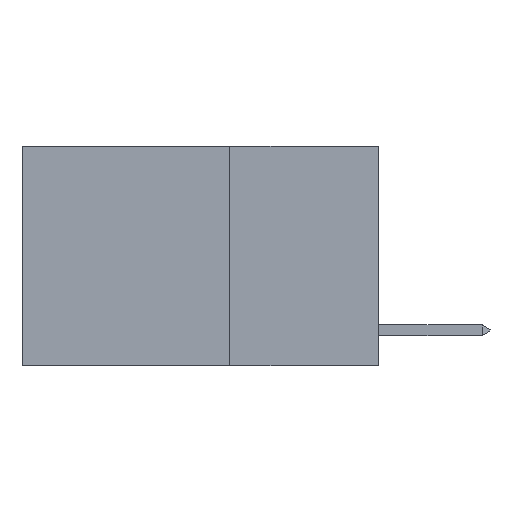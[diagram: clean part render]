
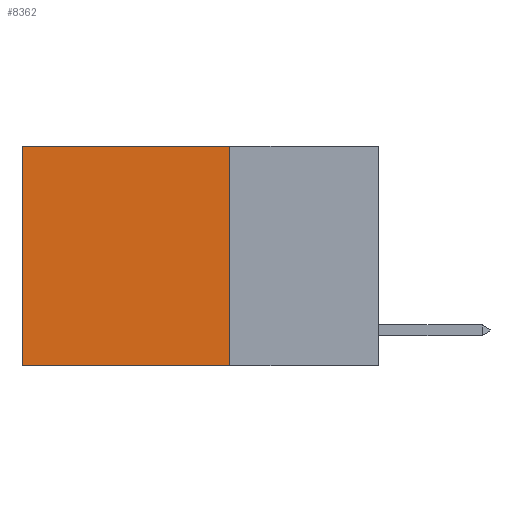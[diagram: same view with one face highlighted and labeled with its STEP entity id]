
A CAD part, left-side view. The second image highlights one B-rep face of the part: STEP entity #8362.
In plain terms, the highlighted planar face has unit normal (-1, 0, 0).
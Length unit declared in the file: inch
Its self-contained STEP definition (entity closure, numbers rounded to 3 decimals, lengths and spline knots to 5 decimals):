
#175 = VECTOR ( 'NONE', #8512, 39.37008 ) ;
#304 = EDGE_CURVE ( 'NONE', #1968, #10467, #11217, .T. ) ;
#358 = ORIENTED_EDGE ( 'NONE', *, *, #304, .F. ) ;
#713 = ORIENTED_EDGE ( 'NONE', *, *, #8503, .F. ) ;
#1292 = EDGE_CURVE ( 'NONE', #1968, #9118, #7324, .T. ) ;
#1561 = CARTESIAN_POINT ( 'NONE',  ( 0.2625, 0.25, -0.37 ) ) ;
#1917 = CARTESIAN_POINT ( 'NONE',  ( 0.2625, 0.25, 0. ) ) ;
#1968 = VERTEX_POINT ( 'NONE', #3652 ) ;
#2159 = DIRECTION ( 'NONE',  ( 0., 1., 0. ) ) ;
#2371 = VECTOR ( 'NONE', #3181, 39.37008 ) ;
#2618 = VECTOR ( 'NONE', #2159, 39.37008 ) ;
#2633 = ORIENTED_EDGE ( 'NONE', *, *, #3169, .T. ) ;
#2778 = LINE ( 'NONE', #3753, #175 ) ;
#3169 = EDGE_CURVE ( 'NONE', #9118, #8665, #2778, .T. ) ;
#3181 = DIRECTION ( 'NONE',  ( 0., 1., 0. ) ) ;
#3652 = CARTESIAN_POINT ( 'NONE',  ( 0.2625, 0.25, 0. ) ) ;
#3753 = CARTESIAN_POINT ( 'NONE',  ( 0.2625, 0.6, 0. ) ) ;
#4064 = CARTESIAN_POINT ( 'NONE',  ( 0.2625, 0.25, 0. ) ) ;
#4105 = PLANE ( 'NONE',  #7825 ) ;
#4203 = CARTESIAN_POINT ( 'NONE',  ( 0.2625, 0.25, -0.37 ) ) ;
#4768 = EDGE_LOOP ( 'NONE', ( #2633, #713, #358, #6042 ) ) ;
#5844 = DIRECTION ( 'NONE',  ( 1., 0., 0. ) ) ;
#5882 = CARTESIAN_POINT ( 'NONE',  ( 0.2625, 0.6, 0. ) ) ;
#6042 = ORIENTED_EDGE ( 'NONE', *, *, #1292, .T. ) ;
#6413 = FACE_OUTER_BOUND ( 'NONE', #4768, .T. ) ;
#6439 = CARTESIAN_POINT ( 'NONE',  ( 0.2625, 0.6, -0.37 ) ) ;
#6922 = CARTESIAN_POINT ( 'NONE',  ( 0.2625, 0.25, 0. ) ) ;
#6977 = LINE ( 'NONE', #4203, #2371 ) ;
#7324 = LINE ( 'NONE', #6922, #2618 ) ;
#7825 = AXIS2_PLACEMENT_3D ( 'NONE', #1917, #5844, #9645 ) ;
#8362 = ADVANCED_FACE ( 'NONE', ( #6413 ), #4105, .F. ) ;
#8503 = EDGE_CURVE ( 'NONE', #10467, #8665, #6977, .T. ) ;
#8512 = DIRECTION ( 'NONE',  ( 0., 0., -1. ) ) ;
#8665 = VERTEX_POINT ( 'NONE', #6439 ) ;
#9118 = VERTEX_POINT ( 'NONE', #5882 ) ;
#9645 = DIRECTION ( 'NONE',  ( 0., 0., -1. ) ) ;
#10467 = VERTEX_POINT ( 'NONE', #1561 ) ;
#10835 = DIRECTION ( 'NONE',  ( 0., 0., -1. ) ) ;
#11217 = LINE ( 'NONE', #4064, #11798 ) ;
#11798 = VECTOR ( 'NONE', #10835, 39.37008 ) ;
